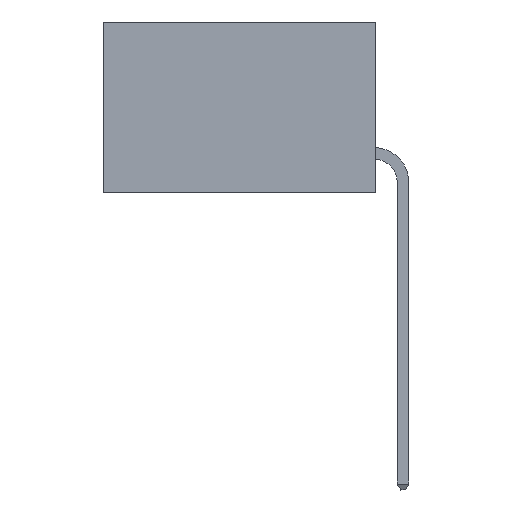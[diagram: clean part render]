
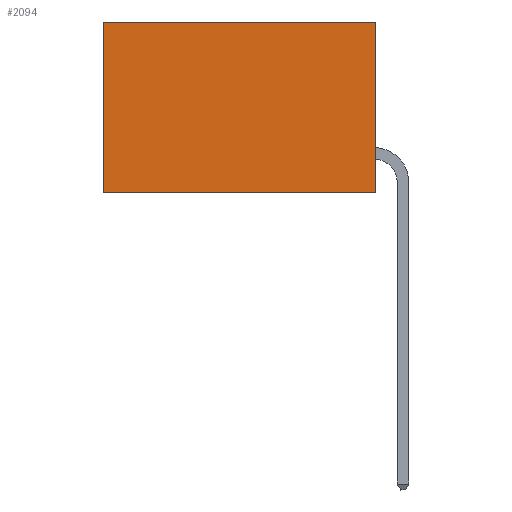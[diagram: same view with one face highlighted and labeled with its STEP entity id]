
A CAD part, left-side view. The second image highlights one B-rep face of the part: STEP entity #2094.
In plain terms, the highlighted planar face has unit normal (-1, 0, 0).
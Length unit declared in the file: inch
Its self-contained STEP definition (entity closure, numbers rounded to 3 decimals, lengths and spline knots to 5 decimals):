
#50 = CARTESIAN_POINT ( 'NONE',  ( 0.277, 0.59, -0.37 ) ) ;
#216 = LINE ( 'NONE', #780, #8287 ) ;
#230 = CARTESIAN_POINT ( 'NONE',  ( 0.277, 0.59, 0. ) ) ;
#259 = VERTEX_POINT ( 'NONE', #4117 ) ;
#732 = DIRECTION ( 'NONE',  ( 0., 1., 0. ) ) ;
#780 = CARTESIAN_POINT ( 'NONE',  ( 0.277, 0., -0.37 ) ) ;
#1289 = DIRECTION ( 'NONE',  ( 0., 1., 0. ) ) ;
#1314 = CARTESIAN_POINT ( 'NONE',  ( 0.277, 0., 0. ) ) ;
#1525 = PLANE ( 'NONE',  #3583 ) ;
#1645 = CARTESIAN_POINT ( 'NONE',  ( 0.277, 0., -0.37 ) ) ;
#1949 = VERTEX_POINT ( 'NONE', #230 ) ;
#1953 = LINE ( 'NONE', #5035, #6272 ) ;
#1962 = VECTOR ( 'NONE', #1289, 39.37008 ) ;
#2094 = ADVANCED_FACE ( 'NONE', ( #5015 ), #1525, .F. ) ;
#3112 = EDGE_CURVE ( 'NONE', #4788, #259, #9557, .T. ) ;
#3315 = VECTOR ( 'NONE', #7260, 39.37008 ) ;
#3583 = AXIS2_PLACEMENT_3D ( 'NONE', #1645, #6152, #7017 ) ;
#3814 = ORIENTED_EDGE ( 'NONE', *, *, #4475, .T. ) ;
#4117 = CARTESIAN_POINT ( 'NONE',  ( 0.277, 0., -0.37 ) ) ;
#4475 = EDGE_CURVE ( 'NONE', #4788, #1949, #6504, .T. ) ;
#4489 = DIRECTION ( 'NONE',  ( 0., 0., -1. ) ) ;
#4788 = VERTEX_POINT ( 'NONE', #8692 ) ;
#4985 = EDGE_CURVE ( 'NONE', #1949, #7744, #1953, .T. ) ;
#5015 = FACE_OUTER_BOUND ( 'NONE', #8229, .T. ) ;
#5035 = CARTESIAN_POINT ( 'NONE',  ( 0.277, 0.59, -0.37 ) ) ;
#6152 = DIRECTION ( 'NONE',  ( 1., 0., 0. ) ) ;
#6232 = ORIENTED_EDGE ( 'NONE', *, *, #6456, .F. ) ;
#6259 = ORIENTED_EDGE ( 'NONE', *, *, #4985, .T. ) ;
#6272 = VECTOR ( 'NONE', #4489, 39.37008 ) ;
#6456 = EDGE_CURVE ( 'NONE', #259, #7744, #216, .T. ) ;
#6504 = LINE ( 'NONE', #1314, #1962 ) ;
#7017 = DIRECTION ( 'NONE',  ( 0., 0., -1. ) ) ;
#7260 = DIRECTION ( 'NONE',  ( 0., 0., -1. ) ) ;
#7397 = CARTESIAN_POINT ( 'NONE',  ( 0.277, 0., -0.37 ) ) ;
#7744 = VERTEX_POINT ( 'NONE', #50 ) ;
#8229 = EDGE_LOOP ( 'NONE', ( #6259, #6232, #10065, #3814 ) ) ;
#8287 = VECTOR ( 'NONE', #732, 39.37008 ) ;
#8692 = CARTESIAN_POINT ( 'NONE',  ( 0.277, 0., 0. ) ) ;
#9557 = LINE ( 'NONE', #7397, #3315 ) ;
#10065 = ORIENTED_EDGE ( 'NONE', *, *, #3112, .F. ) ;
